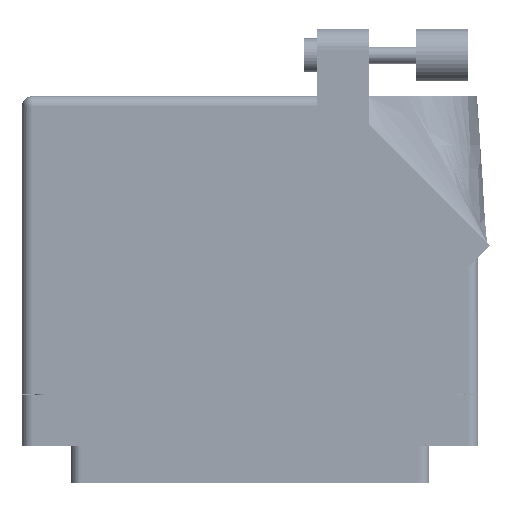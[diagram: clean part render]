
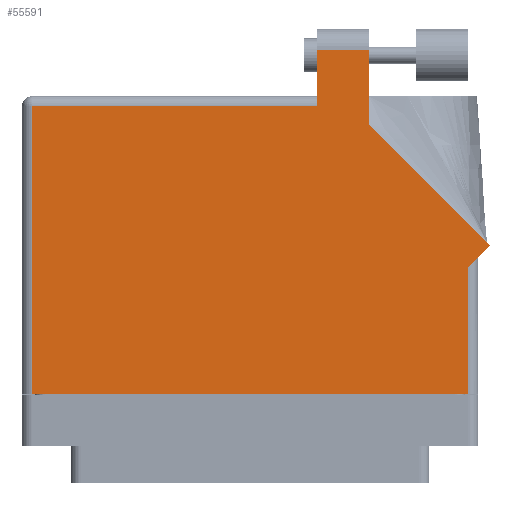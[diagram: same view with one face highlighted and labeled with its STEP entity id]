
A CAD part, front view. The second image highlights one B-rep face of the part: STEP entity #55591.
In plain terms, the highlighted face is planar.
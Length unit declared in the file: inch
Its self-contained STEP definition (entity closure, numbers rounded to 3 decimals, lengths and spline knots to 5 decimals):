
#98 = CARTESIAN_POINT ( 'NONE',  ( -1.359, 1.675, 0.617 ) ) ;
#158 = EDGE_CURVE ( 'NONE', #6041, #64551, #57688, .T. ) ;
#3941 = LINE ( 'NONE', #9730, #23524 ) ;
#4561 = EDGE_CURVE ( 'NONE', #41229, #71616, #37818, .T. ) ;
#4746 = DIRECTION ( 'NONE',  ( 0., 1., 0. ) ) ;
#5124 = DIRECTION ( 'NONE',  ( 0., 0., -1. ) ) ;
#6041 = VERTEX_POINT ( 'NONE', #48817 ) ;
#7147 = CARTESIAN_POINT ( 'NONE',  ( -1.297, 1.613, 0.617 ) ) ;
#7650 = LINE ( 'NONE', #51399, #51382 ) ;
#7742 = EDGE_CURVE ( 'NONE', #64551, #28075, #67635, .T. ) ;
#8803 = EDGE_CURVE ( 'NONE', #65082, #54324, #7650, .T. ) ;
#9730 = CARTESIAN_POINT ( 'NONE',  ( 1.297, 0.715, 0.617 ) ) ;
#11915 = LINE ( 'NONE', #58933, #29821 ) ;
#14629 = CARTESIAN_POINT ( 'NONE',  ( 1.297, -0.1, 0.617 ) ) ;
#15471 = CARTESIAN_POINT ( 'NONE',  ( 0.706, 1.50942, 0.617 ) ) ;
#17188 = DIRECTION ( 'NONE',  ( -0.707, 0.707, 0. ) ) ;
#17761 = ORIENTED_EDGE ( 'NONE', *, *, #7742, .T. ) ;
#19500 = CARTESIAN_POINT ( 'NONE',  ( -1.359, 1.613, 0.617 ) ) ;
#20021 = CARTESIAN_POINT ( 'NONE',  ( 0.706, 1.95, 0.617 ) ) ;
#20107 = ORIENTED_EDGE ( 'NONE', *, *, #53384, .T. ) ;
#20167 = VECTOR ( 'NONE', #47964, 39.37008 ) ;
#20455 = CARTESIAN_POINT ( 'NONE',  ( 0.399, 1.613, 0.617 ) ) ;
#23117 = VERTEX_POINT ( 'NONE', #14629 ) ;
#23524 = VECTOR ( 'NONE', #4746, 39.37008 ) ;
#24376 = VECTOR ( 'NONE', #32353, 39.37008 ) ;
#24600 = EDGE_CURVE ( 'NONE', #54324, #41229, #46795, .T. ) ;
#27776 = DIRECTION ( 'NONE',  ( -1., 0., 0. ) ) ;
#28075 = VERTEX_POINT ( 'NONE', #7147 ) ;
#28169 = CARTESIAN_POINT ( 'NONE',  ( -1.297, -0.1, 0.617 ) ) ;
#28704 = DIRECTION ( 'NONE',  ( 0.707, 0.707, 0. ) ) ;
#29821 = VECTOR ( 'NONE', #64426, 39.37008 ) ;
#31661 = VECTOR ( 'NONE', #17188, 39.37008 ) ;
#32353 = DIRECTION ( 'NONE',  ( -1., 0., 0. ) ) ;
#33176 = DIRECTION ( 'NONE',  ( 0., -1., 0. ) ) ;
#36308 = ORIENTED_EDGE ( 'NONE', *, *, #8803, .T. ) ;
#37818 = LINE ( 'NONE', #65156, #66345 ) ;
#39579 = LINE ( 'NONE', #49033, #24376 ) ;
#41229 = VERTEX_POINT ( 'NONE', #15471 ) ;
#41330 = ORIENTED_EDGE ( 'NONE', *, *, #24600, .T. ) ;
#42207 = CARTESIAN_POINT ( 'NONE',  ( 0.399, 1.675, 0.617 ) ) ;
#42236 = ORIENTED_EDGE ( 'NONE', *, *, #158, .T. ) ;
#46795 = LINE ( 'NONE', #56338, #31661 ) ;
#47964 = DIRECTION ( 'NONE',  ( 0., -1., 0. ) ) ;
#48432 = ORIENTED_EDGE ( 'NONE', *, *, #68679, .T. ) ;
#48817 = CARTESIAN_POINT ( 'NONE',  ( 0.399, 1.95, 0.617 ) ) ;
#49033 = CARTESIAN_POINT ( 'NONE',  ( 0.399, 1.95, 0.617 ) ) ;
#49375 = EDGE_CURVE ( 'NONE', #28075, #65683, #55015, .T. ) ;
#50578 = VECTOR ( 'NONE', #33176, 39.37008 ) ;
#51382 = VECTOR ( 'NONE', #28704, 39.37008 ) ;
#51399 = CARTESIAN_POINT ( 'NONE',  ( 1.359, 0.715, 0.617 ) ) ;
#52185 = EDGE_CURVE ( 'NONE', #65683, #23117, #11915, .T. ) ;
#52454 = VECTOR ( 'NONE', #70872, 39.37008 ) ;
#53384 = EDGE_CURVE ( 'NONE', #71616, #6041, #39579, .T. ) ;
#54324 = VERTEX_POINT ( 'NONE', #55006 ) ;
#54372 = FACE_OUTER_BOUND ( 'NONE', #66329, .T. ) ;
#55006 = CARTESIAN_POINT ( 'NONE',  ( 1.42971, 0.78571, 0.617 ) ) ;
#55015 = LINE ( 'NONE', #61604, #50578 ) ;
#55591 = ADVANCED_FACE ( 'NONE', ( #54372 ), #56245, .F. ) ;
#56245 = PLANE ( 'NONE',  #58087 ) ;
#56338 = CARTESIAN_POINT ( 'NONE',  ( 1.42971, 0.78571, 0.617 ) ) ;
#56381 = ORIENTED_EDGE ( 'NONE', *, *, #49375, .T. ) ;
#57688 = LINE ( 'NONE', #42207, #20167 ) ;
#58087 = AXIS2_PLACEMENT_3D ( 'NONE', #98, #5124, #27776 ) ;
#58933 = CARTESIAN_POINT ( 'NONE',  ( -1.359, -0.1, 0.617 ) ) ;
#61604 = CARTESIAN_POINT ( 'NONE',  ( -1.297, -0.1, 0.617 ) ) ;
#62832 = ORIENTED_EDGE ( 'NONE', *, *, #4561, .T. ) ;
#63726 = CARTESIAN_POINT ( 'NONE',  ( 1.297, 0.653, 0.617 ) ) ;
#64426 = DIRECTION ( 'NONE',  ( 1., 0., 0. ) ) ;
#64551 = VERTEX_POINT ( 'NONE', #20455 ) ;
#65082 = VERTEX_POINT ( 'NONE', #63726 ) ;
#65156 = CARTESIAN_POINT ( 'NONE',  ( 0.706, 1.50942, 0.617 ) ) ;
#65683 = VERTEX_POINT ( 'NONE', #28169 ) ;
#66329 = EDGE_LOOP ( 'NONE', ( #62832, #20107, #42236, #17761, #56381, #68691, #48432, #36308, #41330 ) ) ;
#66345 = VECTOR ( 'NONE', #70867, 39.37008 ) ;
#67635 = LINE ( 'NONE', #19500, #52454 ) ;
#68679 = EDGE_CURVE ( 'NONE', #23117, #65082, #3941, .T. ) ;
#68691 = ORIENTED_EDGE ( 'NONE', *, *, #52185, .T. ) ;
#70867 = DIRECTION ( 'NONE',  ( 0., 1., 0. ) ) ;
#70872 = DIRECTION ( 'NONE',  ( -1., 0., 0. ) ) ;
#71616 = VERTEX_POINT ( 'NONE', #20021 ) ;
